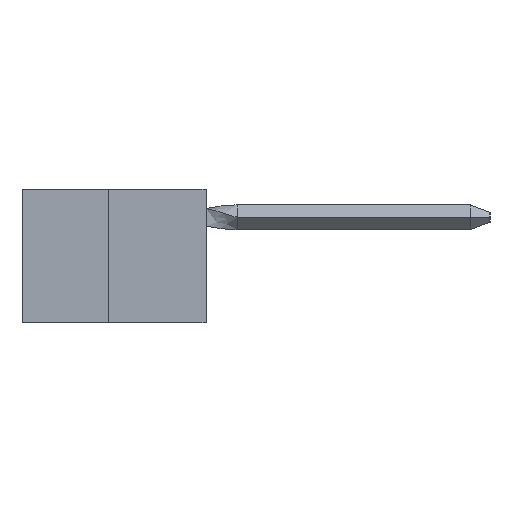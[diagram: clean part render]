
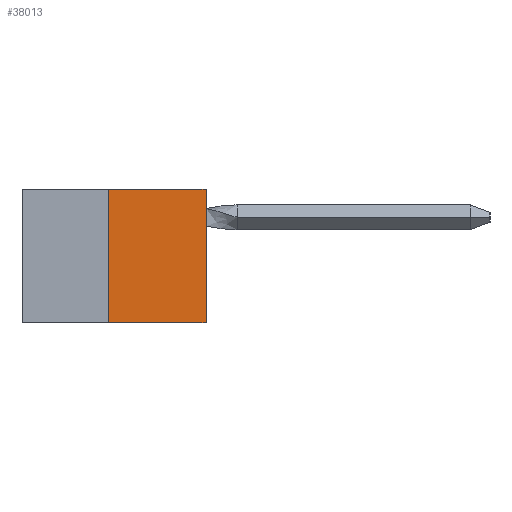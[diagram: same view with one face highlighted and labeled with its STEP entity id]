
A CAD part, left-side view. The second image highlights one B-rep face of the part: STEP entity #38013.
In plain terms, the highlighted planar face has unit normal (-1, 0, 0).
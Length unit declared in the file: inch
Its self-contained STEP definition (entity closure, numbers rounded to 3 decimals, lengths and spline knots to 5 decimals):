
#3488 = LINE ( 'NONE', #35268, #5118 ) ;
#3612 = LINE ( 'NONE', #18434, #26047 ) ;
#3656 = CARTESIAN_POINT ( 'NONE',  ( 0., 0.473, -0.343 ) ) ;
#4612 = DIRECTION ( 'NONE',  ( 0., -1., 0. ) ) ;
#5118 = VECTOR ( 'NONE', #42004, 39.37008 ) ;
#5660 = EDGE_CURVE ( 'NONE', #22515, #23683, #25244, .T. ) ;
#6876 = DIRECTION ( 'NONE',  ( 0., -1., 0. ) ) ;
#8201 = FACE_OUTER_BOUND ( 'NONE', #43791, .T. ) ;
#9092 = EDGE_CURVE ( 'NONE', #22515, #19473, #10656, .T. ) ;
#10325 = CARTESIAN_POINT ( 'NONE',  ( 0., 0., 0. ) ) ;
#10656 = LINE ( 'NONE', #16368, #39606 ) ;
#10893 = PLANE ( 'NONE',  #19999 ) ;
#12128 = CARTESIAN_POINT ( 'NONE',  ( 0., 0.25, -0.343 ) ) ;
#16368 = CARTESIAN_POINT ( 'NONE',  ( 0., 0.25, 0. ) ) ;
#16801 = VERTEX_POINT ( 'NONE', #10325 ) ;
#17017 = EDGE_CURVE ( 'NONE', #19473, #16801, #3612, .T. ) ;
#18434 = CARTESIAN_POINT ( 'NONE',  ( 0., 0.473, 0. ) ) ;
#19273 = DIRECTION ( 'NONE',  ( 0., 0., 1. ) ) ;
#19473 = VERTEX_POINT ( 'NONE', #24401 ) ;
#19999 = AXIS2_PLACEMENT_3D ( 'NONE', #25102, #39474, #35804 ) ;
#22460 = ORIENTED_EDGE ( 'NONE', *, *, #5660, .T. ) ;
#22515 = VERTEX_POINT ( 'NONE', #12128 ) ;
#23683 = VERTEX_POINT ( 'NONE', #43390 ) ;
#24149 = VECTOR ( 'NONE', #6876, 39.37008 ) ;
#24401 = CARTESIAN_POINT ( 'NONE',  ( 0., 0.25, 0. ) ) ;
#25102 = CARTESIAN_POINT ( 'NONE',  ( 0., 0.473, 0. ) ) ;
#25244 = LINE ( 'NONE', #3656, #24149 ) ;
#26047 = VECTOR ( 'NONE', #4612, 39.37008 ) ;
#26626 = EDGE_CURVE ( 'NONE', #23683, #16801, #3488, .T. ) ;
#27109 = ORIENTED_EDGE ( 'NONE', *, *, #17017, .F. ) ;
#29216 = ORIENTED_EDGE ( 'NONE', *, *, #26626, .T. ) ;
#35268 = CARTESIAN_POINT ( 'NONE',  ( 0., 0., 0. ) ) ;
#35804 = DIRECTION ( 'NONE',  ( 0., 0., -1. ) ) ;
#36847 = ORIENTED_EDGE ( 'NONE', *, *, #9092, .F. ) ;
#38013 = ADVANCED_FACE ( 'NONE', ( #8201 ), #10893, .F. ) ;
#39474 = DIRECTION ( 'NONE',  ( 1., 0., 0. ) ) ;
#39606 = VECTOR ( 'NONE', #19273, 39.37008 ) ;
#42004 = DIRECTION ( 'NONE',  ( 0., 0., 1. ) ) ;
#43390 = CARTESIAN_POINT ( 'NONE',  ( 0., 0., -0.343 ) ) ;
#43791 = EDGE_LOOP ( 'NONE', ( #27109, #36847, #22460, #29216 ) ) ;
